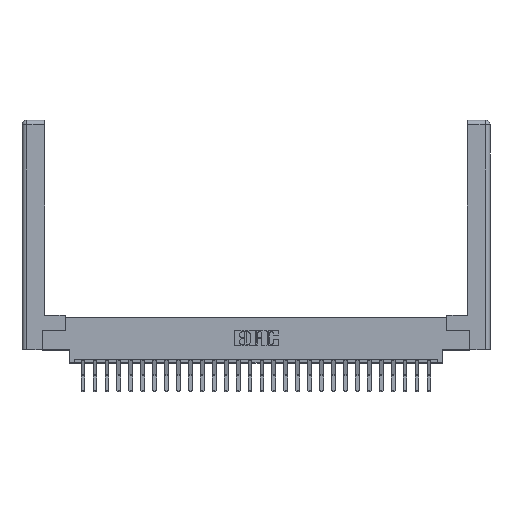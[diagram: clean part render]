
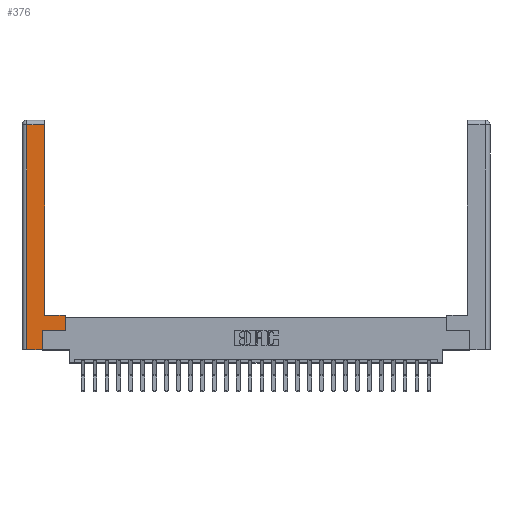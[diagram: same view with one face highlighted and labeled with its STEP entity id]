
A CAD part, top view. The second image highlights one B-rep face of the part: STEP entity #376.
In plain terms, the highlighted planar face has unit normal (0, 0, 1).
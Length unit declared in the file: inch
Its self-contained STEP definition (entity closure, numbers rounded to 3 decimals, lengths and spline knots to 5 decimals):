
#183 = VERTEX_POINT ( 'NONE', #16298 ) ;
#376 = ADVANCED_FACE ( 'NONE', ( #10334 ), #17926, .F. ) ;
#459 = ORIENTED_EDGE ( 'NONE', *, *, #5629, .T. ) ;
#1196 = LINE ( 'NONE', #15409, #25984 ) ;
#2718 = CARTESIAN_POINT ( 'NONE',  ( 0.295, 0.45, 0. ) ) ;
#3558 = DIRECTION ( 'NONE',  ( 0., 1., 0. ) ) ;
#4167 = ORIENTED_EDGE ( 'NONE', *, *, #26286, .T. ) ;
#4490 = CARTESIAN_POINT ( 'NONE',  ( 0.565, 0.245, 0. ) ) ;
#4632 = VECTOR ( 'NONE', #5145, 39.37008 ) ;
#5145 = DIRECTION ( 'NONE',  ( 0., 1., 0. ) ) ;
#5284 = CARTESIAN_POINT ( 'NONE',  ( 0.265, 0.245, 0. ) ) ;
#5629 = EDGE_CURVE ( 'NONE', #7147, #19656, #27011, .T. ) ;
#5795 = VERTEX_POINT ( 'NONE', #7253 ) ;
#6446 = VERTEX_POINT ( 'NONE', #16785 ) ;
#6618 = DIRECTION ( 'NONE',  ( -1., 0., 0. ) ) ;
#7147 = VERTEX_POINT ( 'NONE', #25246 ) ;
#7253 = CARTESIAN_POINT ( 'NONE',  ( 0.265, 0.245, 0. ) ) ;
#7259 = VECTOR ( 'NONE', #15448, 39.37008 ) ;
#7293 = ORIENTED_EDGE ( 'NONE', *, *, #21727, .T. ) ;
#7485 = VERTEX_POINT ( 'NONE', #11181 ) ;
#8780 = DIRECTION ( 'NONE',  ( 1., 0., 0. ) ) ;
#9305 = LINE ( 'NONE', #24346, #4632 ) ;
#9395 = DIRECTION ( 'NONE',  ( -1., 0., 0. ) ) ;
#10334 = FACE_OUTER_BOUND ( 'NONE', #22995, .T. ) ;
#11181 = CARTESIAN_POINT ( 'NONE',  ( 0.0615, 2.94, 0. ) ) ;
#11254 = DIRECTION ( 'NONE',  ( 1., 0., 0. ) ) ;
#11421 = DIRECTION ( 'NONE',  ( 0., 0., -1. ) ) ;
#12950 = CARTESIAN_POINT ( 'NONE',  ( 0.295, 2.94, 0. ) ) ;
#13305 = CARTESIAN_POINT ( 'NONE',  ( 0.0615, 2.94, 0. ) ) ;
#13321 = EDGE_CURVE ( 'NONE', #5795, #6446, #18139, .T. ) ;
#13450 = DIRECTION ( 'NONE',  ( 0., -1., 0. ) ) ;
#13508 = VECTOR ( 'NONE', #8780, 39.37008 ) ;
#14055 = VERTEX_POINT ( 'NONE', #14860 ) ;
#14860 = CARTESIAN_POINT ( 'NONE',  ( 0.0615, 0., 0. ) ) ;
#15076 = VECTOR ( 'NONE', #3558, 39.37008 ) ;
#15409 = CARTESIAN_POINT ( 'NONE',  ( 0.0615, 0., 0. ) ) ;
#15448 = DIRECTION ( 'NONE',  ( -1., 0., 0. ) ) ;
#15715 = CARTESIAN_POINT ( 'NONE',  ( 0., 0., 0. ) ) ;
#16157 = VECTOR ( 'NONE', #11254, 39.37008 ) ;
#16298 = CARTESIAN_POINT ( 'NONE',  ( 0.265, 0., 0. ) ) ;
#16785 = CARTESIAN_POINT ( 'NONE',  ( 0.565, 0.245, 0. ) ) ;
#17011 = CARTESIAN_POINT ( 'NONE',  ( 0.295, 0.45, 0. ) ) ;
#17311 = CARTESIAN_POINT ( 'NONE',  ( 0.265, 0., 0. ) ) ;
#17926 = PLANE ( 'NONE',  #21196 ) ;
#18139 = LINE ( 'NONE', #4490, #16157 ) ;
#18162 = LINE ( 'NONE', #13305, #23505 ) ;
#18828 = VECTOR ( 'NONE', #20265, 39.37008 ) ;
#18932 = ORIENTED_EDGE ( 'NONE', *, *, #22307, .T. ) ;
#19656 = VERTEX_POINT ( 'NONE', #17011 ) ;
#20221 = EDGE_CURVE ( 'NONE', #14055, #183, #22836, .T. ) ;
#20265 = DIRECTION ( 'NONE',  ( 0., 1., 0. ) ) ;
#20718 = LINE ( 'NONE', #24977, #15076 ) ;
#21196 = AXIS2_PLACEMENT_3D ( 'NONE', #15715, #11421, #9395 ) ;
#21727 = EDGE_CURVE ( 'NONE', #6446, #7147, #20718, .T. ) ;
#21833 = LINE ( 'NONE', #5284, #18828 ) ;
#22307 = EDGE_CURVE ( 'NONE', #19656, #26829, #9305, .T. ) ;
#22836 = LINE ( 'NONE', #17311, #13508 ) ;
#22995 = EDGE_LOOP ( 'NONE', ( #18932, #4167, #26869, #24552, #23530, #23112, #7293, #459 ) ) ;
#23112 = ORIENTED_EDGE ( 'NONE', *, *, #13321, .T. ) ;
#23505 = VECTOR ( 'NONE', #6618, 39.37008 ) ;
#23530 = ORIENTED_EDGE ( 'NONE', *, *, #27674, .T. ) ;
#24346 = CARTESIAN_POINT ( 'NONE',  ( 0.295, 3., 0. ) ) ;
#24352 = EDGE_CURVE ( 'NONE', #7485, #14055, #1196, .T. ) ;
#24552 = ORIENTED_EDGE ( 'NONE', *, *, #20221, .T. ) ;
#24977 = CARTESIAN_POINT ( 'NONE',  ( 0.565, 0.45, 0. ) ) ;
#25246 = CARTESIAN_POINT ( 'NONE',  ( 0.565, 0.45, 0. ) ) ;
#25984 = VECTOR ( 'NONE', #13450, 39.37008 ) ;
#26286 = EDGE_CURVE ( 'NONE', #26829, #7485, #18162, .T. ) ;
#26829 = VERTEX_POINT ( 'NONE', #12950 ) ;
#26869 = ORIENTED_EDGE ( 'NONE', *, *, #24352, .T. ) ;
#27011 = LINE ( 'NONE', #2718, #7259 ) ;
#27674 = EDGE_CURVE ( 'NONE', #183, #5795, #21833, .T. ) ;
